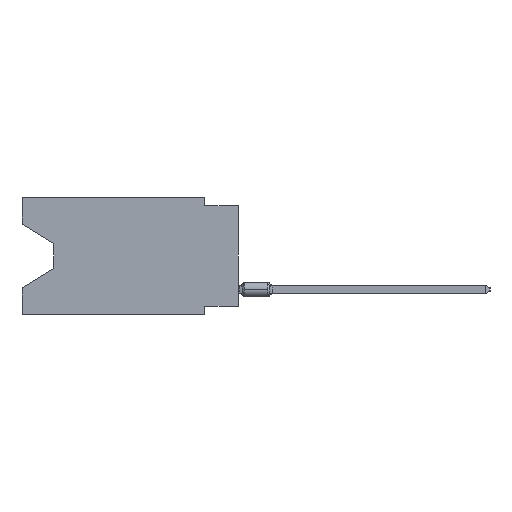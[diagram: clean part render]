
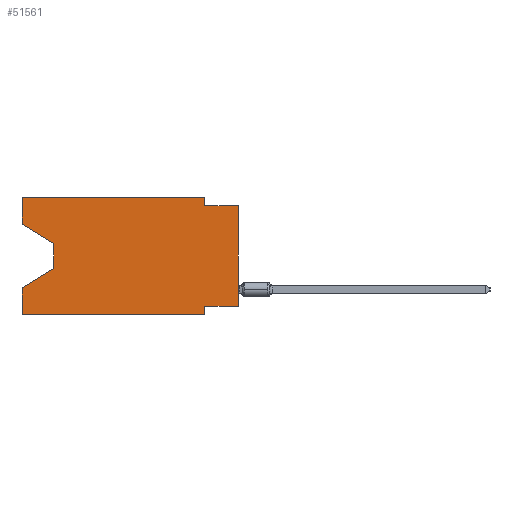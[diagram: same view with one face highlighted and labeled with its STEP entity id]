
A CAD part, left-side view. The second image highlights one B-rep face of the part: STEP entity #51561.
In plain terms, the highlighted planar face has unit normal (-1, 0, 0).
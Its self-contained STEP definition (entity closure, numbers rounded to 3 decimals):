
#732 = ORIENTED_EDGE ( 'NONE', *, *, #49055, .T. ) ;
#746 = VECTOR ( 'NONE', #50134, 1000. ) ;
#1134 = PLANE ( 'NONE',  #42337 ) ;
#2815 = DIRECTION ( 'NONE',  ( 0., 0.855, -0.519 ) ) ;
#3225 = DIRECTION ( 'NONE',  ( 0., 0., 1. ) ) ;
#4044 = CARTESIAN_POINT ( 'NONE',  ( 0., 0., 0. ) ) ;
#4131 = VERTEX_POINT ( 'NONE', #40560 ) ;
#4269 = VECTOR ( 'NONE', #3225, 1000. ) ;
#4478 = CARTESIAN_POINT ( 'NONE',  ( 0., 13.97, -3.505 ) ) ;
#5908 = VERTEX_POINT ( 'NONE', #31660 ) ;
#7005 = EDGE_CURVE ( 'NONE', #27429, #46974, #39148, .T. ) ;
#7759 = ORIENTED_EDGE ( 'NONE', *, *, #7005, .F. ) ;
#8579 = LINE ( 'NONE', #41837, #4269 ) ;
#10287 = ORIENTED_EDGE ( 'NONE', *, *, #43272, .F. ) ;
#10494 = DIRECTION ( 'NONE',  ( 0., 0., -1. ) ) ;
#12009 = LINE ( 'NONE', #46111, #28792 ) ;
#12353 = CARTESIAN_POINT ( 'NONE',  ( 0., 16.383, 0. ) ) ;
#12525 = EDGE_CURVE ( 'NONE', #45690, #27429, #27467, .T. ) ;
#12637 = LINE ( 'NONE', #39398, #37672 ) ;
#13205 = VECTOR ( 'NONE', #46209, 1000. ) ;
#13238 = CARTESIAN_POINT ( 'NONE',  ( 0., 16.383, -2.038 ) ) ;
#13620 = LINE ( 'NONE', #4044, #49367 ) ;
#13747 = DIRECTION ( 'NONE',  ( 0., -1., 0. ) ) ;
#13931 = VECTOR ( 'NONE', #21956, 1000. ) ;
#14294 = VERTEX_POINT ( 'NONE', #13238 ) ;
#14659 = FACE_OUTER_BOUND ( 'NONE', #38024, .T. ) ;
#15159 = CARTESIAN_POINT ( 'NONE',  ( 0., 16.383, -2.038 ) ) ;
#15221 = VERTEX_POINT ( 'NONE', #50431 ) ;
#15521 = CARTESIAN_POINT ( 'NONE',  ( 0., 13.97, -3.505 ) ) ;
#16991 = CARTESIAN_POINT ( 'NONE',  ( 0., 2.54, -0.635 ) ) ;
#17424 = EDGE_CURVE ( 'NONE', #14294, #45690, #8579, .T. ) ;
#18159 = VERTEX_POINT ( 'NONE', #28468 ) ;
#18330 = CARTESIAN_POINT ( 'NONE',  ( 0., 16.383, 0. ) ) ;
#21956 = DIRECTION ( 'NONE',  ( 0., 0., -1. ) ) ;
#22613 = EDGE_CURVE ( 'NONE', #24978, #15221, #12009, .T. ) ;
#23237 = CARTESIAN_POINT ( 'NONE',  ( 0., 16.383, 0. ) ) ;
#24548 = LINE ( 'NONE', #15521, #51551 ) ;
#24770 = LINE ( 'NONE', #55466, #746 ) ;
#24978 = VERTEX_POINT ( 'NONE', #26040 ) ;
#25834 = CARTESIAN_POINT ( 'NONE',  ( 0., 2.54, 0. ) ) ;
#25845 = CARTESIAN_POINT ( 'NONE',  ( 0., 2.54, -8.255 ) ) ;
#26040 = CARTESIAN_POINT ( 'NONE',  ( 0., 16.383, -8.89 ) ) ;
#26702 = EDGE_CURVE ( 'NONE', #18159, #5908, #13620, .T. ) ;
#27429 = VERTEX_POINT ( 'NONE', #25834 ) ;
#27467 = LINE ( 'NONE', #23237, #50085 ) ;
#28468 = CARTESIAN_POINT ( 'NONE',  ( 0., 0., -8.255 ) ) ;
#28792 = VECTOR ( 'NONE', #50912, 1000. ) ;
#29065 = VERTEX_POINT ( 'NONE', #48551 ) ;
#30003 = DIRECTION ( 'NONE',  ( 0., 0., -1. ) ) ;
#30702 = ORIENTED_EDGE ( 'NONE', *, *, #26702, .T. ) ;
#30842 = LINE ( 'NONE', #51993, #49086 ) ;
#31660 = CARTESIAN_POINT ( 'NONE',  ( 0., 0., -0.635 ) ) ;
#31731 = ORIENTED_EDGE ( 'NONE', *, *, #37005, .F. ) ;
#32106 = ORIENTED_EDGE ( 'NONE', *, *, #53935, .T. ) ;
#32687 = LINE ( 'NONE', #54678, #47449 ) ;
#33264 = LINE ( 'NONE', #55211, #13205 ) ;
#33759 = VECTOR ( 'NONE', #45047, 1000. ) ;
#34815 = ORIENTED_EDGE ( 'NONE', *, *, #12525, .F. ) ;
#35526 = DIRECTION ( 'NONE',  ( 0., 0., -1. ) ) ;
#36567 = LINE ( 'NONE', #15159, #33759 ) ;
#37005 = EDGE_CURVE ( 'NONE', #18159, #38936, #33264, .T. ) ;
#37007 = EDGE_CURVE ( 'NONE', #4131, #15221, #32687, .T. ) ;
#37672 = VECTOR ( 'NONE', #13747, 1000. ) ;
#38024 = EDGE_LOOP ( 'NONE', ( #46553, #32106, #49819, #52226, #732, #10287, #31731, #30702, #43602, #7759, #34815, #47996 ) ) ;
#38936 = VERTEX_POINT ( 'NONE', #25845 ) ;
#39148 = LINE ( 'NONE', #43661, #13931 ) ;
#39398 = CARTESIAN_POINT ( 'NONE',  ( 0., 0., -0.635 ) ) ;
#39786 = EDGE_CURVE ( 'NONE', #14294, #50598, #36567, .T. ) ;
#40420 = DIRECTION ( 'NONE',  ( 0., -1., 0. ) ) ;
#40560 = CARTESIAN_POINT ( 'NONE',  ( 0., 13.97, -5.385 ) ) ;
#41837 = CARTESIAN_POINT ( 'NONE',  ( 0., 16.383, 0. ) ) ;
#42337 = AXIS2_PLACEMENT_3D ( 'NONE', #18330, #49334, #35526 ) ;
#43272 = EDGE_CURVE ( 'NONE', #38936, #29065, #30842, .T. ) ;
#43602 = ORIENTED_EDGE ( 'NONE', *, *, #47949, .F. ) ;
#43661 = CARTESIAN_POINT ( 'NONE',  ( 0., 2.54, 0. ) ) ;
#45047 = DIRECTION ( 'NONE',  ( 0., -0.855, -0.519 ) ) ;
#45690 = VERTEX_POINT ( 'NONE', #12353 ) ;
#46111 = CARTESIAN_POINT ( 'NONE',  ( 0., 16.383, 0. ) ) ;
#46209 = DIRECTION ( 'NONE',  ( 0., 1., 0. ) ) ;
#46553 = ORIENTED_EDGE ( 'NONE', *, *, #39786, .T. ) ;
#46974 = VERTEX_POINT ( 'NONE', #16991 ) ;
#47449 = VECTOR ( 'NONE', #2815, 1000. ) ;
#47454 = DIRECTION ( 'NONE',  ( 0., 0., 1. ) ) ;
#47949 = EDGE_CURVE ( 'NONE', #46974, #5908, #12637, .T. ) ;
#47996 = ORIENTED_EDGE ( 'NONE', *, *, #17424, .F. ) ;
#48551 = CARTESIAN_POINT ( 'NONE',  ( 0., 2.54, -8.89 ) ) ;
#49055 = EDGE_CURVE ( 'NONE', #24978, #29065, #24770, .T. ) ;
#49086 = VECTOR ( 'NONE', #30003, 1000. ) ;
#49334 = DIRECTION ( 'NONE',  ( 1., 0., 0. ) ) ;
#49367 = VECTOR ( 'NONE', #47454, 1000. ) ;
#49819 = ORIENTED_EDGE ( 'NONE', *, *, #37007, .T. ) ;
#50085 = VECTOR ( 'NONE', #40420, 1000. ) ;
#50134 = DIRECTION ( 'NONE',  ( 0., -1., 0. ) ) ;
#50431 = CARTESIAN_POINT ( 'NONE',  ( 0., 16.383, -6.852 ) ) ;
#50598 = VERTEX_POINT ( 'NONE', #4478 ) ;
#50912 = DIRECTION ( 'NONE',  ( 0., 0., 1. ) ) ;
#51551 = VECTOR ( 'NONE', #10494, 1000. ) ;
#51561 = ADVANCED_FACE ( 'NONE', ( #14659 ), #1134, .F. ) ;
#51993 = CARTESIAN_POINT ( 'NONE',  ( 0., 2.54, -8.89 ) ) ;
#52226 = ORIENTED_EDGE ( 'NONE', *, *, #22613, .F. ) ;
#53935 = EDGE_CURVE ( 'NONE', #50598, #4131, #24548, .T. ) ;
#54678 = CARTESIAN_POINT ( 'NONE',  ( 0., 13.97, -5.385 ) ) ;
#55211 = CARTESIAN_POINT ( 'NONE',  ( 0., 0., -8.255 ) ) ;
#55466 = CARTESIAN_POINT ( 'NONE',  ( 0., 16.383, -8.89 ) ) ;
